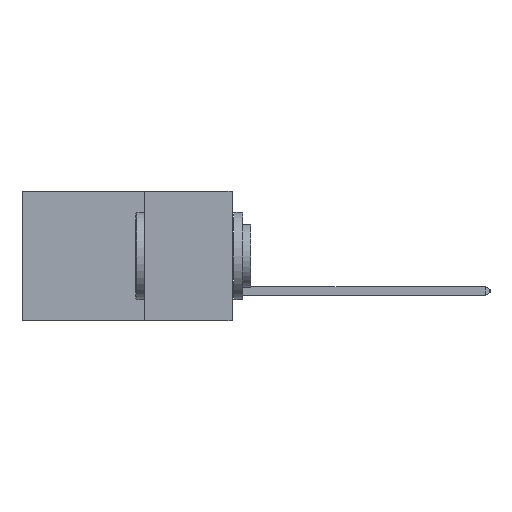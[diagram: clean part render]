
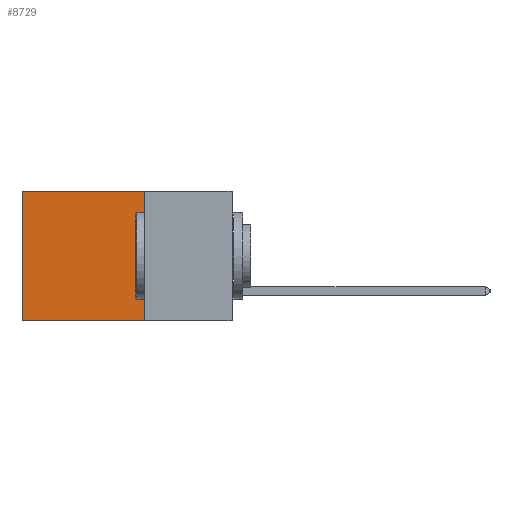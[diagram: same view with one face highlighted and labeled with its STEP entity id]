
A CAD part, left-side view. The second image highlights one B-rep face of the part: STEP entity #8729.
In plain terms, the highlighted planar face has unit normal (-1, 0, 0).
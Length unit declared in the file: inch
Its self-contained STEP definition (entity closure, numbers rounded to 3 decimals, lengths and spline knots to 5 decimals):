
#35 = PLANE ( 'NONE',  #12173 ) ;
#299 = ORIENTED_EDGE ( 'NONE', *, *, #13616, .F. ) ;
#402 = CARTESIAN_POINT ( 'NONE',  ( 0.2875, 0.6, 0. ) ) ;
#2953 = CARTESIAN_POINT ( 'NONE',  ( 0.2875, 0.25, 0. ) ) ;
#3237 = DIRECTION ( 'NONE',  ( 0., 0., -1. ) ) ;
#3322 = CARTESIAN_POINT ( 'NONE',  ( 0.2875, 0.6, 0. ) ) ;
#4089 = CARTESIAN_POINT ( 'NONE',  ( 0.2875, 0.25, 0. ) ) ;
#4473 = CARTESIAN_POINT ( 'NONE',  ( 0.2875, 0.6, -0.37 ) ) ;
#5147 = ORIENTED_EDGE ( 'NONE', *, *, #23625, .T. ) ;
#5765 = DIRECTION ( 'NONE',  ( 0., 0., -1. ) ) ;
#5890 = VERTEX_POINT ( 'NONE', #8832 ) ;
#6116 = DIRECTION ( 'NONE',  ( 0., 0., -1. ) ) ;
#7581 = VERTEX_POINT ( 'NONE', #4473 ) ;
#7964 = EDGE_CURVE ( 'NONE', #24029, #5890, #8047, .T. ) ;
#8047 = LINE ( 'NONE', #17694, #22753 ) ;
#8729 = ADVANCED_FACE ( 'NONE', ( #21430 ), #35, .F. ) ;
#8832 = CARTESIAN_POINT ( 'NONE',  ( 0.2875, 0.25, -0.37 ) ) ;
#9511 = VECTOR ( 'NONE', #25744, 39.37008 ) ;
#11632 = EDGE_CURVE ( 'NONE', #14834, #7581, #21192, .T. ) ;
#12173 = AXIS2_PLACEMENT_3D ( 'NONE', #4089, #18041, #6116 ) ;
#13267 = ORIENTED_EDGE ( 'NONE', *, *, #11632, .T. ) ;
#13616 = EDGE_CURVE ( 'NONE', #5890, #7581, #24813, .T. ) ;
#13684 = CARTESIAN_POINT ( 'NONE',  ( 0.2875, 0.25, 0. ) ) ;
#14217 = LINE ( 'NONE', #13684, #24875 ) ;
#14834 = VERTEX_POINT ( 'NONE', #402 ) ;
#15691 = DIRECTION ( 'NONE',  ( 0., 1., 0. ) ) ;
#16272 = EDGE_LOOP ( 'NONE', ( #13267, #299, #23486, #5147 ) ) ;
#17694 = CARTESIAN_POINT ( 'NONE',  ( 0.2875, 0.25, 0. ) ) ;
#18041 = DIRECTION ( 'NONE',  ( 1., 0., 0. ) ) ;
#21192 = LINE ( 'NONE', #3322, #25852 ) ;
#21430 = FACE_OUTER_BOUND ( 'NONE', #16272, .T. ) ;
#22753 = VECTOR ( 'NONE', #5765, 39.37008 ) ;
#23486 = ORIENTED_EDGE ( 'NONE', *, *, #7964, .F. ) ;
#23625 = EDGE_CURVE ( 'NONE', #24029, #14834, #14217, .T. ) ;
#23771 = CARTESIAN_POINT ( 'NONE',  ( 0.2875, 0.25, -0.37 ) ) ;
#24029 = VERTEX_POINT ( 'NONE', #2953 ) ;
#24813 = LINE ( 'NONE', #23771, #9511 ) ;
#24875 = VECTOR ( 'NONE', #15691, 39.37008 ) ;
#25744 = DIRECTION ( 'NONE',  ( 0., 1., 0. ) ) ;
#25852 = VECTOR ( 'NONE', #3237, 39.37008 ) ;
